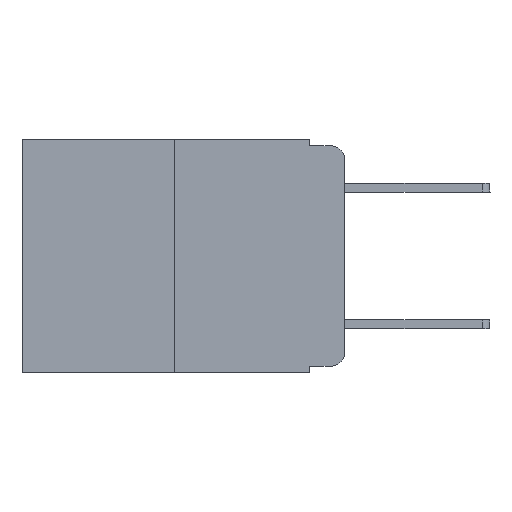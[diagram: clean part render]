
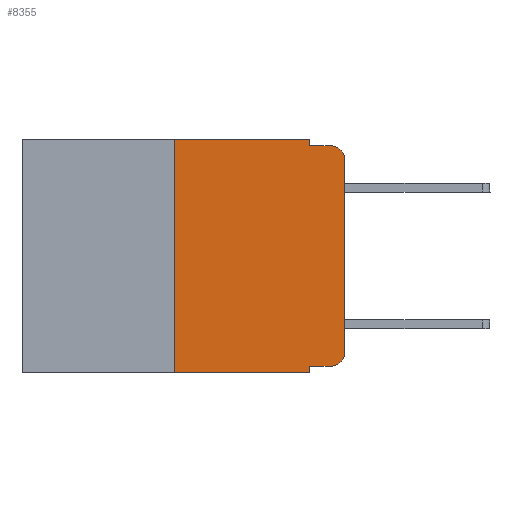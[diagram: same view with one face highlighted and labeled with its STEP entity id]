
A CAD part, left-side view. The second image highlights one B-rep face of the part: STEP entity #8355.
In plain terms, the highlighted planar face has unit normal (-1, 0, 0).
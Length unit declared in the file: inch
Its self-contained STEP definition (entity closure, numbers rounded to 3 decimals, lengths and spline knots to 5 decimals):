
#202 = LINE ( 'NONE', #6033, #18676 ) ;
#271 = DIRECTION ( 'NONE',  ( -1., 0., 0. ) ) ;
#468 = CARTESIAN_POINT ( 'NONE',  ( 0., 0.051, 0. ) ) ;
#472 = DIRECTION ( 'NONE',  ( 0., 0., -1. ) ) ;
#505 = CARTESIAN_POINT ( 'NONE',  ( 0., 0.25, -0.343 ) ) ;
#617 = VERTEX_POINT ( 'NONE', #18562 ) ;
#929 = DIRECTION ( 'NONE',  ( 0., 0., 1. ) ) ;
#1533 = VERTEX_POINT ( 'NONE', #7248 ) ;
#1684 = EDGE_CURVE ( 'NONE', #617, #5690, #7342, .T. ) ;
#1799 = DIRECTION ( 'NONE',  ( 0., 0., -1. ) ) ;
#2070 = CARTESIAN_POINT ( 'NONE',  ( 0., 0.25, 0. ) ) ;
#2805 = CARTESIAN_POINT ( 'NONE',  ( 0., 0.473, -0.343 ) ) ;
#2934 = DIRECTION ( 'NONE',  ( 0., -1., 0. ) ) ;
#3037 = CARTESIAN_POINT ( 'NONE',  ( 0., 0.02, -0.01 ) ) ;
#4517 = VECTOR ( 'NONE', #14116, 39.37008 ) ;
#4983 = CARTESIAN_POINT ( 'NONE',  ( 0., 0., 0. ) ) ;
#5028 = VERTEX_POINT ( 'NONE', #12253 ) ;
#5171 = LINE ( 'NONE', #4983, #4517 ) ;
#5507 = EDGE_CURVE ( 'NONE', #6443, #5028, #5171, .T. ) ;
#5690 = VERTEX_POINT ( 'NONE', #14295 ) ;
#6033 = CARTESIAN_POINT ( 'NONE',  ( 0., 0.473, 0. ) ) ;
#6116 = CARTESIAN_POINT ( 'NONE',  ( 0., 0.051, -0.01 ) ) ;
#6190 = EDGE_CURVE ( 'NONE', #617, #6686, #17532, .T. ) ;
#6268 = EDGE_LOOP ( 'NONE', ( #6522, #10924, #18074, #15281, #18492, #17367, #7393, #8663, #13625, #14514 ) ) ;
#6443 = VERTEX_POINT ( 'NONE', #7046 ) ;
#6522 = ORIENTED_EDGE ( 'NONE', *, *, #5507, .T. ) ;
#6668 = EDGE_CURVE ( 'NONE', #12916, #7343, #7319, .T. ) ;
#6686 = VERTEX_POINT ( 'NONE', #17599 ) ;
#7046 = CARTESIAN_POINT ( 'NONE',  ( 0., 0., -0.313 ) ) ;
#7248 = CARTESIAN_POINT ( 'NONE',  ( 0., 0.25, 0. ) ) ;
#7292 = AXIS2_PLACEMENT_3D ( 'NONE', #10334, #13617, #472 ) ;
#7319 = LINE ( 'NONE', #14828, #11321 ) ;
#7342 = LINE ( 'NONE', #468, #9686 ) ;
#7343 = VERTEX_POINT ( 'NONE', #10046 ) ;
#7347 = DIRECTION ( 'NONE',  ( 0., 0., -1. ) ) ;
#7393 = ORIENTED_EDGE ( 'NONE', *, *, #12324, .T. ) ;
#7515 = EDGE_CURVE ( 'NONE', #5028, #18812, #15570, .T. ) ;
#7591 = EDGE_CURVE ( 'NONE', #15364, #1533, #12260, .T. ) ;
#7725 = CARTESIAN_POINT ( 'NONE',  ( 0., 0.02, -0.313 ) ) ;
#8355 = ADVANCED_FACE ( 'NONE', ( #13638 ), #14967, .F. ) ;
#8469 = EDGE_CURVE ( 'NONE', #1533, #12916, #202, .T. ) ;
#8655 = DIRECTION ( 'NONE',  ( 0., -1., 0. ) ) ;
#8663 = ORIENTED_EDGE ( 'NONE', *, *, #1684, .F. ) ;
#8919 = DIRECTION ( 'NONE',  ( 1., 0., 0. ) ) ;
#8927 = AXIS2_PLACEMENT_3D ( 'NONE', #7725, #271, #7347 ) ;
#9005 = LINE ( 'NONE', #6116, #12102 ) ;
#9686 = VECTOR ( 'NONE', #1799, 39.37008 ) ;
#9835 = CIRCLE ( 'NONE', #8927, 0.02 ) ;
#10046 = CARTESIAN_POINT ( 'NONE',  ( 0., 0.051, -0.01 ) ) ;
#10305 = EDGE_CURVE ( 'NONE', #6686, #6443, #9835, .T. ) ;
#10334 = CARTESIAN_POINT ( 'NONE',  ( 0., 0.02, -0.03 ) ) ;
#10633 = DIRECTION ( 'NONE',  ( 0., -1., 0. ) ) ;
#10924 = ORIENTED_EDGE ( 'NONE', *, *, #7515, .T. ) ;
#11321 = VECTOR ( 'NONE', #13208, 39.37008 ) ;
#11904 = DIRECTION ( 'NONE',  ( 0., -1., 0. ) ) ;
#12102 = VECTOR ( 'NONE', #10633, 39.37008 ) ;
#12253 = CARTESIAN_POINT ( 'NONE',  ( 0., 0., -0.03 ) ) ;
#12260 = LINE ( 'NONE', #2070, #15015 ) ;
#12324 = EDGE_CURVE ( 'NONE', #15364, #5690, #12910, .T. ) ;
#12910 = LINE ( 'NONE', #2805, #14509 ) ;
#12916 = VERTEX_POINT ( 'NONE', #15902 ) ;
#13208 = DIRECTION ( 'NONE',  ( 0., 0., -1. ) ) ;
#13617 = DIRECTION ( 'NONE',  ( -1., 0., 0. ) ) ;
#13625 = ORIENTED_EDGE ( 'NONE', *, *, #6190, .T. ) ;
#13638 = FACE_OUTER_BOUND ( 'NONE', #6268, .T. ) ;
#14116 = DIRECTION ( 'NONE',  ( 0., 0., 1. ) ) ;
#14295 = CARTESIAN_POINT ( 'NONE',  ( 0., 0.051, -0.343 ) ) ;
#14414 = EDGE_CURVE ( 'NONE', #7343, #18812, #9005, .T. ) ;
#14509 = VECTOR ( 'NONE', #8655, 39.37008 ) ;
#14514 = ORIENTED_EDGE ( 'NONE', *, *, #10305, .T. ) ;
#14828 = CARTESIAN_POINT ( 'NONE',  ( 0., 0.051, 0. ) ) ;
#14967 = PLANE ( 'NONE',  #15001 ) ;
#15001 = AXIS2_PLACEMENT_3D ( 'NONE', #16206, #8919, #16113 ) ;
#15015 = VECTOR ( 'NONE', #929, 39.37008 ) ;
#15281 = ORIENTED_EDGE ( 'NONE', *, *, #6668, .F. ) ;
#15364 = VERTEX_POINT ( 'NONE', #505 ) ;
#15570 = CIRCLE ( 'NONE', #7292, 0.02 ) ;
#15902 = CARTESIAN_POINT ( 'NONE',  ( 0., 0.051, 0. ) ) ;
#16090 = CARTESIAN_POINT ( 'NONE',  ( 0., 0.051, -0.333 ) ) ;
#16113 = DIRECTION ( 'NONE',  ( 0., 0., -1. ) ) ;
#16198 = VECTOR ( 'NONE', #2934, 39.37008 ) ;
#16206 = CARTESIAN_POINT ( 'NONE',  ( 0., 0.473, 0. ) ) ;
#17367 = ORIENTED_EDGE ( 'NONE', *, *, #7591, .F. ) ;
#17532 = LINE ( 'NONE', #16090, #16198 ) ;
#17599 = CARTESIAN_POINT ( 'NONE',  ( 0., 0.02, -0.333 ) ) ;
#18074 = ORIENTED_EDGE ( 'NONE', *, *, #14414, .F. ) ;
#18492 = ORIENTED_EDGE ( 'NONE', *, *, #8469, .F. ) ;
#18562 = CARTESIAN_POINT ( 'NONE',  ( 0., 0.051, -0.333 ) ) ;
#18676 = VECTOR ( 'NONE', #11904, 39.37008 ) ;
#18812 = VERTEX_POINT ( 'NONE', #3037 ) ;
